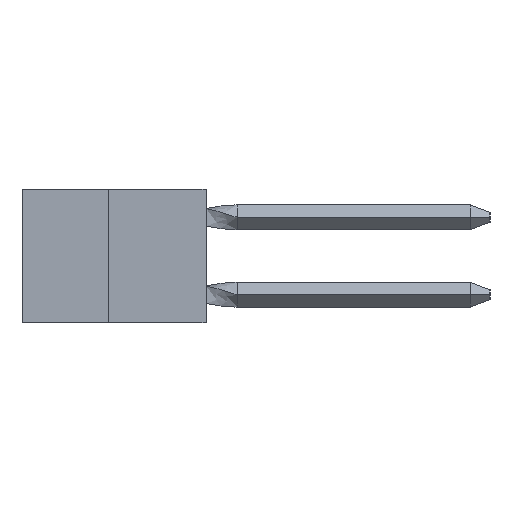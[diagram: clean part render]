
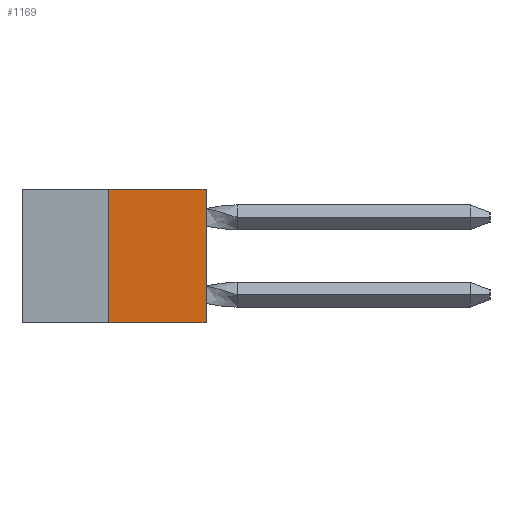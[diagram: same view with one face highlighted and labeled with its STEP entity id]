
A CAD part, left-side view. The second image highlights one B-rep face of the part: STEP entity #1169.
In plain terms, the highlighted planar face has unit normal (-1, 0, 0).
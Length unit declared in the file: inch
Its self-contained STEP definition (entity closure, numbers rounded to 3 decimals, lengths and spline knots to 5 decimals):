
#733 = CARTESIAN_POINT ( 'NONE',  ( 0., 0.473, 0. ) ) ;
#1169 = ADVANCED_FACE ( 'NONE', ( #10980 ), #29505, .F. ) ;
#1950 = ORIENTED_EDGE ( 'NONE', *, *, #10737, .F. ) ;
#6459 = DIRECTION ( 'NONE',  ( 0., 0., 1. ) ) ;
#6583 = CARTESIAN_POINT ( 'NONE',  ( 0., 0.25, 0. ) ) ;
#7581 = CARTESIAN_POINT ( 'NONE',  ( 0., 0.473, -0.343 ) ) ;
#7883 = CARTESIAN_POINT ( 'NONE',  ( 0., 0.473, 0. ) ) ;
#9597 = VECTOR ( 'NONE', #6459, 39.37008 ) ;
#10737 = EDGE_CURVE ( 'NONE', #10977, #28574, #25004, .T. ) ;
#10936 = EDGE_LOOP ( 'NONE', ( #27806, #1950, #21465, #22295 ) ) ;
#10977 = VERTEX_POINT ( 'NONE', #23169 ) ;
#10980 = FACE_OUTER_BOUND ( 'NONE', #10936, .T. ) ;
#12400 = LINE ( 'NONE', #7883, #17372 ) ;
#12659 = CARTESIAN_POINT ( 'NONE',  ( 0., 0.25, 0. ) ) ;
#16701 = CARTESIAN_POINT ( 'NONE',  ( 0., 0., -0.343 ) ) ;
#17372 = VECTOR ( 'NONE', #19655, 39.37008 ) ;
#19219 = AXIS2_PLACEMENT_3D ( 'NONE', #733, #35476, #20761 ) ;
#19655 = DIRECTION ( 'NONE',  ( 0., -1., 0. ) ) ;
#20761 = DIRECTION ( 'NONE',  ( 0., 0., -1. ) ) ;
#21465 = ORIENTED_EDGE ( 'NONE', *, *, #26322, .T. ) ;
#22295 = ORIENTED_EDGE ( 'NONE', *, *, #31857, .T. ) ;
#22559 = DIRECTION ( 'NONE',  ( 0., 0., 1. ) ) ;
#22885 = VERTEX_POINT ( 'NONE', #16701 ) ;
#23169 = CARTESIAN_POINT ( 'NONE',  ( 0., 0.25, -0.343 ) ) ;
#25004 = LINE ( 'NONE', #6583, #9597 ) ;
#25078 = VERTEX_POINT ( 'NONE', #29850 ) ;
#26322 = EDGE_CURVE ( 'NONE', #10977, #22885, #33364, .T. ) ;
#27038 = EDGE_CURVE ( 'NONE', #28574, #25078, #12400, .T. ) ;
#27218 = LINE ( 'NONE', #36927, #29472 ) ;
#27806 = ORIENTED_EDGE ( 'NONE', *, *, #27038, .F. ) ;
#28574 = VERTEX_POINT ( 'NONE', #12659 ) ;
#29472 = VECTOR ( 'NONE', #22559, 39.37008 ) ;
#29505 = PLANE ( 'NONE',  #19219 ) ;
#29673 = VECTOR ( 'NONE', #36389, 39.37008 ) ;
#29850 = CARTESIAN_POINT ( 'NONE',  ( 0., 0., 0. ) ) ;
#31857 = EDGE_CURVE ( 'NONE', #22885, #25078, #27218, .T. ) ;
#33364 = LINE ( 'NONE', #7581, #29673 ) ;
#35476 = DIRECTION ( 'NONE',  ( 1., 0., 0. ) ) ;
#36389 = DIRECTION ( 'NONE',  ( 0., -1., 0. ) ) ;
#36927 = CARTESIAN_POINT ( 'NONE',  ( 0., 0., 0. ) ) ;
